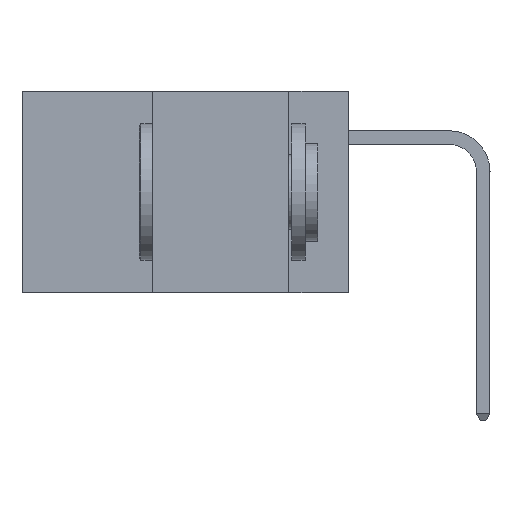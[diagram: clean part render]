
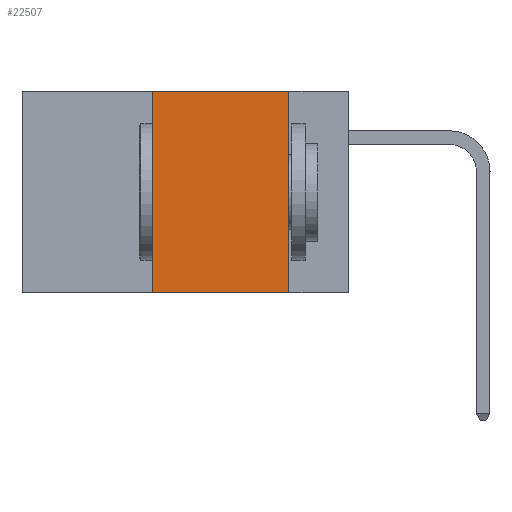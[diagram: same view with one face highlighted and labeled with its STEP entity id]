
A CAD part, left-side view. The second image highlights one B-rep face of the part: STEP entity #22507.
In plain terms, the highlighted planar face has unit normal (-1, 0, 0).
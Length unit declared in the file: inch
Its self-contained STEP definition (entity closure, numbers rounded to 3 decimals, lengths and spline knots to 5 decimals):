
#956 = DIRECTION ( 'NONE',  ( 0., -1., 0. ) ) ;
#1587 = ORIENTED_EDGE ( 'NONE', *, *, #16392, .F. ) ;
#2381 = VECTOR ( 'NONE', #6995, 39.37008 ) ;
#2450 = DIRECTION ( 'NONE',  ( 0., 0., -1. ) ) ;
#2718 = CARTESIAN_POINT ( 'NONE',  ( 0., 0.36, 0. ) ) ;
#3768 = VECTOR ( 'NONE', #23024, 39.37008 ) ;
#4879 = CARTESIAN_POINT ( 'NONE',  ( 0., 0.11, -0.37 ) ) ;
#5234 = FACE_OUTER_BOUND ( 'NONE', #24955, .T. ) ;
#6643 = CARTESIAN_POINT ( 'NONE',  ( 0., 0.6, -0.37 ) ) ;
#6750 = EDGE_CURVE ( 'NONE', #19276, #19108, #11654, .T. ) ;
#6995 = DIRECTION ( 'NONE',  ( 0., -1., 0. ) ) ;
#7792 = CARTESIAN_POINT ( 'NONE',  ( 0., 0.36, 0. ) ) ;
#9074 = CARTESIAN_POINT ( 'NONE',  ( 0., 0.11, 0. ) ) ;
#9508 = AXIS2_PLACEMENT_3D ( 'NONE', #12160, #14059, #2450 ) ;
#10194 = PLANE ( 'NONE',  #9508 ) ;
#11034 = VECTOR ( 'NONE', #23896, 39.37008 ) ;
#11552 = CARTESIAN_POINT ( 'NONE',  ( 0., 0.11, 0. ) ) ;
#11654 = LINE ( 'NONE', #2718, #11034 ) ;
#12160 = CARTESIAN_POINT ( 'NONE',  ( 0., 0.6, 0. ) ) ;
#14059 = DIRECTION ( 'NONE',  ( 1., 0., 0. ) ) ;
#14078 = LINE ( 'NONE', #11552, #3768 ) ;
#14893 = VERTEX_POINT ( 'NONE', #4879 ) ;
#15830 = EDGE_CURVE ( 'NONE', #24204, #14893, #14078, .T. ) ;
#16392 = EDGE_CURVE ( 'NONE', #19108, #24204, #22301, .T. ) ;
#18540 = VECTOR ( 'NONE', #956, 39.37008 ) ;
#19038 = ORIENTED_EDGE ( 'NONE', *, *, #6750, .F. ) ;
#19108 = VERTEX_POINT ( 'NONE', #7792 ) ;
#19276 = VERTEX_POINT ( 'NONE', #19516 ) ;
#19354 = ORIENTED_EDGE ( 'NONE', *, *, #15830, .F. ) ;
#19516 = CARTESIAN_POINT ( 'NONE',  ( 0., 0.36, -0.37 ) ) ;
#20194 = EDGE_CURVE ( 'NONE', #19276, #14893, #24251, .T. ) ;
#20762 = ORIENTED_EDGE ( 'NONE', *, *, #20194, .T. ) ;
#22301 = LINE ( 'NONE', #22412, #2381 ) ;
#22412 = CARTESIAN_POINT ( 'NONE',  ( 0., 0.6, 0. ) ) ;
#22507 = ADVANCED_FACE ( 'NONE', ( #5234 ), #10194, .F. ) ;
#23024 = DIRECTION ( 'NONE',  ( 0., 0., -1. ) ) ;
#23896 = DIRECTION ( 'NONE',  ( 0., 0., 1. ) ) ;
#24204 = VERTEX_POINT ( 'NONE', #9074 ) ;
#24251 = LINE ( 'NONE', #6643, #18540 ) ;
#24955 = EDGE_LOOP ( 'NONE', ( #19354, #1587, #19038, #20762 ) ) ;
